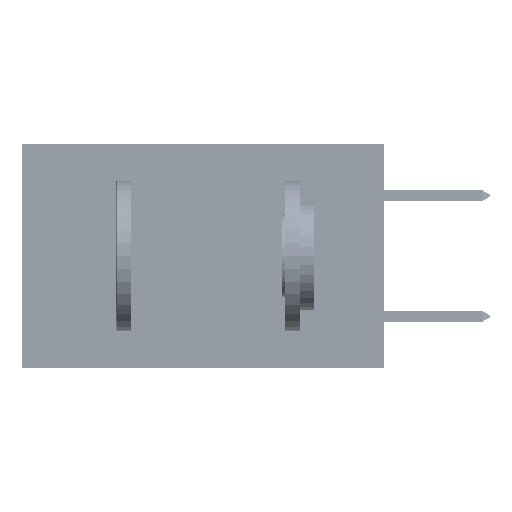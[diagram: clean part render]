
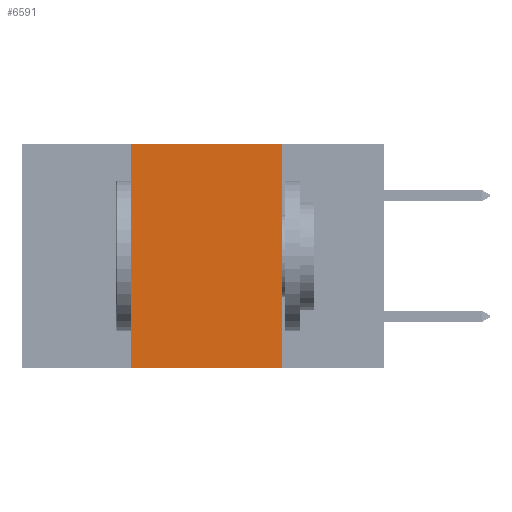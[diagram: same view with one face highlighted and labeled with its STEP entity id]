
A CAD part, left-side view. The second image highlights one B-rep face of the part: STEP entity #6591.
In plain terms, the highlighted planar face has unit normal (-1, 0, 0).
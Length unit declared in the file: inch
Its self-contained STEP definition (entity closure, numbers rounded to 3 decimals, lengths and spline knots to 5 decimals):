
#1010 = AXIS2_PLACEMENT_3D ( 'NONE', #45160, #5500, #26411 ) ;
#2466 = DIRECTION ( 'NONE',  ( 0., 0., -1. ) ) ;
#2576 = LINE ( 'NONE', #16466, #21475 ) ;
#3024 = VERTEX_POINT ( 'NONE', #36159 ) ;
#3340 = CARTESIAN_POINT ( 'NONE',  ( 0., 0.42, 0. ) ) ;
#5500 = DIRECTION ( 'NONE',  ( 1., 0., 0. ) ) ;
#6591 = ADVANCED_FACE ( 'NONE', ( #45323 ), #18770, .F. ) ;
#7548 = LINE ( 'NONE', #43873, #46442 ) ;
#8138 = VERTEX_POINT ( 'NONE', #31695 ) ;
#11350 = VERTEX_POINT ( 'NONE', #28738 ) ;
#11370 = EDGE_CURVE ( 'NONE', #3024, #8138, #7548, .T. ) ;
#13692 = DIRECTION ( 'NONE',  ( 0., -1., 0. ) ) ;
#15352 = ORIENTED_EDGE ( 'NONE', *, *, #35768, .F. ) ;
#16466 = CARTESIAN_POINT ( 'NONE',  ( 0., 0.6, 0. ) ) ;
#16525 = ORIENTED_EDGE ( 'NONE', *, *, #45156, .F. ) ;
#17703 = EDGE_LOOP ( 'NONE', ( #43067, #15352, #16525, #28987 ) ) ;
#18770 = PLANE ( 'NONE',  #1010 ) ;
#19753 = CARTESIAN_POINT ( 'NONE',  ( 0., 0.42, -0.37 ) ) ;
#21475 = VECTOR ( 'NONE', #46619, 39.37008 ) ;
#26411 = DIRECTION ( 'NONE',  ( 0., 0., -1. ) ) ;
#28738 = CARTESIAN_POINT ( 'NONE',  ( 0., 0.42, 0. ) ) ;
#28987 = ORIENTED_EDGE ( 'NONE', *, *, #32553, .T. ) ;
#29762 = DIRECTION ( 'NONE',  ( 0., 0., 1. ) ) ;
#31695 = CARTESIAN_POINT ( 'NONE',  ( 0., 0.17, -0.37 ) ) ;
#32180 = CARTESIAN_POINT ( 'NONE',  ( 0., 0.6, -0.37 ) ) ;
#32553 = EDGE_CURVE ( 'NONE', #40281, #8138, #47805, .T. ) ;
#35768 = EDGE_CURVE ( 'NONE', #11350, #3024, #2576, .T. ) ;
#36159 = CARTESIAN_POINT ( 'NONE',  ( 0., 0.17, 0. ) ) ;
#36750 = VECTOR ( 'NONE', #29762, 39.37008 ) ;
#37756 = VECTOR ( 'NONE', #13692, 39.37008 ) ;
#40281 = VERTEX_POINT ( 'NONE', #19753 ) ;
#43067 = ORIENTED_EDGE ( 'NONE', *, *, #11370, .F. ) ;
#43873 = CARTESIAN_POINT ( 'NONE',  ( 0., 0.17, 0. ) ) ;
#45156 = EDGE_CURVE ( 'NONE', #40281, #11350, #45562, .T. ) ;
#45160 = CARTESIAN_POINT ( 'NONE',  ( 0., 0.6, 0. ) ) ;
#45323 = FACE_OUTER_BOUND ( 'NONE', #17703, .T. ) ;
#45562 = LINE ( 'NONE', #3340, #36750 ) ;
#46442 = VECTOR ( 'NONE', #2466, 39.37008 ) ;
#46619 = DIRECTION ( 'NONE',  ( 0., -1., 0. ) ) ;
#47805 = LINE ( 'NONE', #32180, #37756 ) ;
